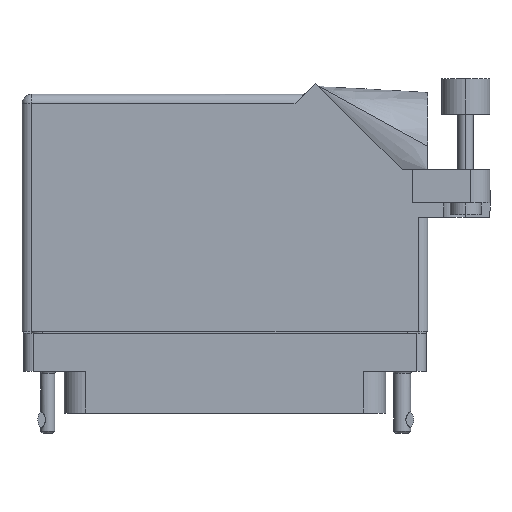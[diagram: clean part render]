
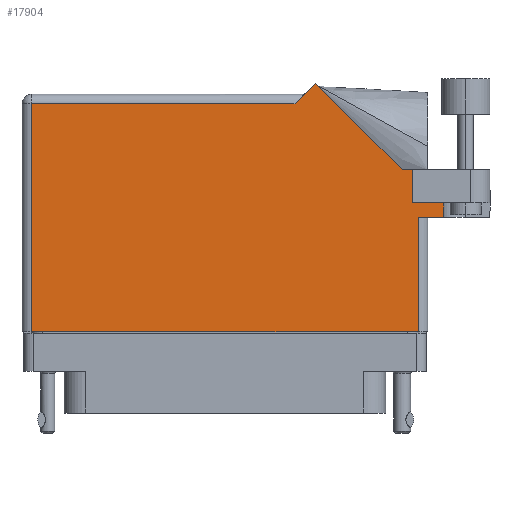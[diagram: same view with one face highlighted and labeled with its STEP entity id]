
A CAD part, front view. The second image highlights one B-rep face of the part: STEP entity #17904.
In plain terms, the highlighted face is planar.
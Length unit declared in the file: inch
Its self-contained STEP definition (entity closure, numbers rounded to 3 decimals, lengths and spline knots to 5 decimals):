
#159 = CARTESIAN_POINT ( 'NONE',  ( 1.14042, 0.944, 0.455 ) ) ;
#252 = LINE ( 'NONE', #54185, #45587 ) ;
#486 = CARTESIAN_POINT ( 'NONE',  ( 1.4075, 0.637, 0.455 ) ) ;
#800 = DIRECTION ( 'NONE',  ( 0., -1., 0. ) ) ;
#2597 = EDGE_CURVE ( 'NONE', #3071, #36014, #4270, .T. ) ;
#3071 = VERTEX_POINT ( 'NONE', #19860 ) ;
#3758 = EDGE_CURVE ( 'NONE', #19106, #41025, #26911, .T. ) ;
#4270 = LINE ( 'NONE', #37120, #32422 ) ;
#4326 = ORIENTED_EDGE ( 'NONE', *, *, #17992, .T. ) ;
#5034 = DIRECTION ( 'NONE',  ( 1., 0., 0. ) ) ;
#5969 = LINE ( 'NONE', #25078, #42493 ) ;
#5985 = DIRECTION ( 'NONE',  ( 0., 1., 0. ) ) ;
#7166 = CARTESIAN_POINT ( 'NONE',  ( 1.4075, 1.06177, 0.455 ) ) ;
#7565 = ORIENTED_EDGE ( 'NONE', *, *, #17115, .F. ) ;
#7708 = EDGE_CURVE ( 'NONE', #40678, #8473, #48802, .T. ) ;
#8473 = VERTEX_POINT ( 'NONE', #21479 ) ;
#8671 = CARTESIAN_POINT ( 'NONE',  ( 1.4075, 0.731, 0.455 ) ) ;
#9103 = LINE ( 'NONE', #20066, #14652 ) ;
#11078 = VERTEX_POINT ( 'NONE', #159 ) ;
#11213 = DIRECTION ( 'NONE',  ( -1., 0., 0. ) ) ;
#11323 = CARTESIAN_POINT ( 'NONE',  ( -1.244, -0.1, 0.455 ) ) ;
#11833 = LINE ( 'NONE', #34643, #13255 ) ;
#11916 = VERTEX_POINT ( 'NONE', #29734 ) ;
#13255 = VECTOR ( 'NONE', #21923, 39.37008 ) ;
#13324 = CARTESIAN_POINT ( 'NONE',  ( 1.306, 0.637, 0.455 ) ) ;
#13673 = VECTOR ( 'NONE', #48011, 39.37008 ) ;
#13831 = CARTESIAN_POINT ( 'NONE',  ( -1.306, -0.1, 0.455 ) ) ;
#14652 = VECTOR ( 'NONE', #37547, 39.37008 ) ;
#14894 = ORIENTED_EDGE ( 'NONE', *, *, #7708, .T. ) ;
#15174 = DIRECTION ( 'NONE',  ( 0., 1., 0. ) ) ;
#16294 = LINE ( 'NONE', #13831, #30770 ) ;
#16812 = CARTESIAN_POINT ( 'NONE',  ( 1.244, 0.637, 0.455 ) ) ;
#17115 = EDGE_CURVE ( 'NONE', #22475, #46015, #38401, .T. ) ;
#17382 = ORIENTED_EDGE ( 'NONE', *, *, #2597, .T. ) ;
#17904 = ADVANCED_FACE ( 'NONE', ( #47984 ), #34666, .F. ) ;
#17992 = EDGE_CURVE ( 'NONE', #41025, #3071, #16294, .T. ) ;
#18635 = DIRECTION ( 'NONE',  ( 1., 0., 0. ) ) ;
#19106 = VERTEX_POINT ( 'NONE', #34851 ) ;
#19860 = CARTESIAN_POINT ( 'NONE',  ( 1.244, -0.1, 0.455 ) ) ;
#20066 = CARTESIAN_POINT ( 'NONE',  ( 1.14042, 0.944, 0.455 ) ) ;
#20296 = DIRECTION ( 'NONE',  ( 0., -1., 0. ) ) ;
#20367 = EDGE_CURVE ( 'NONE', #8473, #19106, #11833, .T. ) ;
#20531 = VECTOR ( 'NONE', #800, 39.37008 ) ;
#20613 = EDGE_CURVE ( 'NONE', #11916, #22475, #252, .T. ) ;
#21479 = CARTESIAN_POINT ( 'NONE',  ( 0.451, 1.368, 0.455 ) ) ;
#21923 = DIRECTION ( 'NONE',  ( -1., 0., 0. ) ) ;
#22475 = VERTEX_POINT ( 'NONE', #8671 ) ;
#22509 = ORIENTED_EDGE ( 'NONE', *, *, #20613, .F. ) ;
#22677 = CARTESIAN_POINT ( 'NONE',  ( 1.206, 0.944, 0.455 ) ) ;
#23146 = EDGE_CURVE ( 'NONE', #11916, #33044, #52707, .T. ) ;
#23262 = ORIENTED_EDGE ( 'NONE', *, *, #23146, .T. ) ;
#24118 = VECTOR ( 'NONE', #20296, 39.37008 ) ;
#24453 = EDGE_CURVE ( 'NONE', #36014, #46015, #44967, .T. ) ;
#25078 = CARTESIAN_POINT ( 'NONE',  ( 1.706, 0.944, 0.455 ) ) ;
#25123 = VECTOR ( 'NONE', #5985, 39.37008 ) ;
#25791 = DIRECTION ( 'NONE',  ( -1., 0., 0. ) ) ;
#26911 = LINE ( 'NONE', #38147, #24118 ) ;
#27493 = ORIENTED_EDGE ( 'NONE', *, *, #3758, .T. ) ;
#29734 = CARTESIAN_POINT ( 'NONE',  ( 1.206, 0.731, 0.455 ) ) ;
#29864 = CARTESIAN_POINT ( 'NONE',  ( 0.58371, 1.50071, 0.455 ) ) ;
#30770 = VECTOR ( 'NONE', #48303, 39.37008 ) ;
#31613 = EDGE_LOOP ( 'NONE', ( #4326, #17382, #36477, #7565, #22509, #23262, #45917, #35523, #14894, #47311, #27493 ) ) ;
#32422 = VECTOR ( 'NONE', #15174, 39.37008 ) ;
#33044 = VERTEX_POINT ( 'NONE', #22677 ) ;
#34643 = CARTESIAN_POINT ( 'NONE',  ( -1.306, 1.368, 0.455 ) ) ;
#34666 = PLANE ( 'NONE',  #52256 ) ;
#34851 = CARTESIAN_POINT ( 'NONE',  ( -1.244, 1.368, 0.455 ) ) ;
#35405 = VECTOR ( 'NONE', #5034, 39.37008 ) ;
#35523 = ORIENTED_EDGE ( 'NONE', *, *, #44143, .T. ) ;
#36014 = VERTEX_POINT ( 'NONE', #16812 ) ;
#36477 = ORIENTED_EDGE ( 'NONE', *, *, #24453, .T. ) ;
#37120 = CARTESIAN_POINT ( 'NONE',  ( 1.244, 0.637, 0.455 ) ) ;
#37547 = DIRECTION ( 'NONE',  ( -0.707, 0.707, 0. ) ) ;
#38147 = CARTESIAN_POINT ( 'NONE',  ( -1.244, -0.1, 0.455 ) ) ;
#38401 = LINE ( 'NONE', #7166, #20531 ) ;
#40678 = VERTEX_POINT ( 'NONE', #29864 ) ;
#41025 = VERTEX_POINT ( 'NONE', #11323 ) ;
#42493 = VECTOR ( 'NONE', #11213, 39.37008 ) ;
#43312 = CARTESIAN_POINT ( 'NONE',  ( -1.306, 1.43, 0.455 ) ) ;
#44143 = EDGE_CURVE ( 'NONE', #11078, #40678, #9103, .T. ) ;
#44967 = LINE ( 'NONE', #13324, #35405 ) ;
#45587 = VECTOR ( 'NONE', #18635, 39.37008 ) ;
#45823 = CARTESIAN_POINT ( 'NONE',  ( 1.206, 0.731, 0.455 ) ) ;
#45917 = ORIENTED_EDGE ( 'NONE', *, *, #48352, .T. ) ;
#46015 = VERTEX_POINT ( 'NONE', #486 ) ;
#47052 = CARTESIAN_POINT ( 'NONE',  ( 0.513, 1.43, 0.455 ) ) ;
#47311 = ORIENTED_EDGE ( 'NONE', *, *, #20367, .T. ) ;
#47729 = DIRECTION ( 'NONE',  ( 0., 0., -1. ) ) ;
#47984 = FACE_OUTER_BOUND ( 'NONE', #31613, .T. ) ;
#48011 = DIRECTION ( 'NONE',  ( -0.707, -0.707, 0. ) ) ;
#48303 = DIRECTION ( 'NONE',  ( 1., 0., 0. ) ) ;
#48352 = EDGE_CURVE ( 'NONE', #33044, #11078, #5969, .T. ) ;
#48802 = LINE ( 'NONE', #47052, #13673 ) ;
#52256 = AXIS2_PLACEMENT_3D ( 'NONE', #43312, #47729, #25791 ) ;
#52707 = LINE ( 'NONE', #45823, #25123 ) ;
#54185 = CARTESIAN_POINT ( 'NONE',  ( 1.206, 0.731, 0.455 ) ) ;
